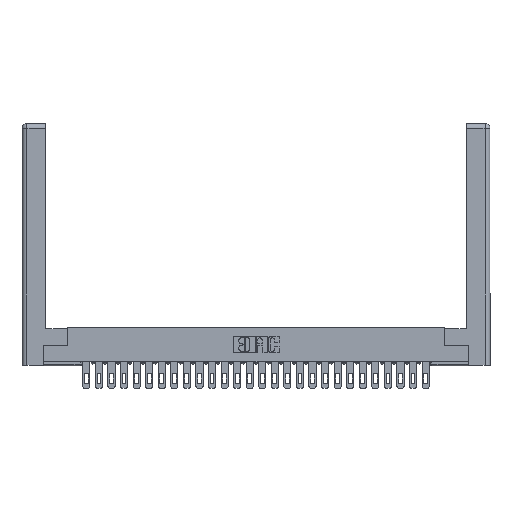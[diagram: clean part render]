
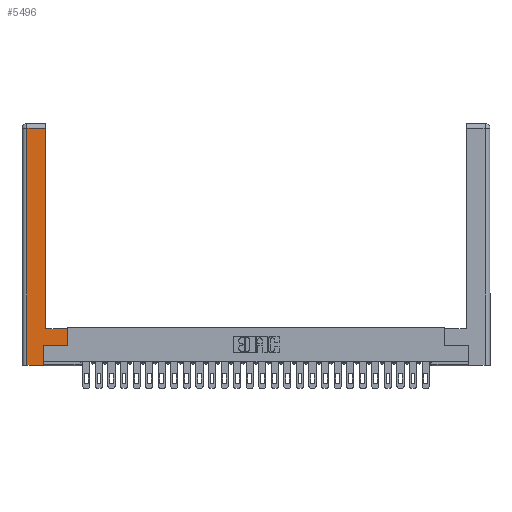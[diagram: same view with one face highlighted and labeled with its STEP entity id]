
A CAD part, top view. The second image highlights one B-rep face of the part: STEP entity #5496.
In plain terms, the highlighted planar face has unit normal (0, 0, 1).
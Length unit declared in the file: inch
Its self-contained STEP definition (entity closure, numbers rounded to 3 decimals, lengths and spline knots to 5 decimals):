
#522 = CARTESIAN_POINT ( 'NONE',  ( 0.295, 2.94, 0. ) ) ;
#1122 = CARTESIAN_POINT ( 'NONE',  ( 0.295, 3., 0. ) ) ;
#1353 = VECTOR ( 'NONE', #4804, 39.37008 ) ;
#2107 = VECTOR ( 'NONE', #16895, 39.37008 ) ;
#3837 = LINE ( 'NONE', #25675, #9139 ) ;
#3874 = PLANE ( 'NONE',  #5296 ) ;
#4760 = CARTESIAN_POINT ( 'NONE',  ( 0.265, 0., 0. ) ) ;
#4804 = DIRECTION ( 'NONE',  ( 0., 1., 0. ) ) ;
#4821 = VERTEX_POINT ( 'NONE', #28256 ) ;
#4866 = EDGE_CURVE ( 'NONE', #8910, #16377, #15898, .T. ) ;
#5296 = AXIS2_PLACEMENT_3D ( 'NONE', #28823, #24265, #22078 ) ;
#5496 = ADVANCED_FACE ( 'NONE', ( #17241 ), #3874, .F. ) ;
#6043 = VERTEX_POINT ( 'NONE', #23443 ) ;
#6126 = ORIENTED_EDGE ( 'NONE', *, *, #4866, .T. ) ;
#7914 = ORIENTED_EDGE ( 'NONE', *, *, #8423, .T. ) ;
#8423 = EDGE_CURVE ( 'NONE', #4821, #15440, #24903, .T. ) ;
#8910 = VERTEX_POINT ( 'NONE', #12033 ) ;
#8972 = LINE ( 'NONE', #1122, #28034 ) ;
#9139 = VECTOR ( 'NONE', #23198, 39.37008 ) ;
#9192 = VERTEX_POINT ( 'NONE', #15165 ) ;
#9513 = LINE ( 'NONE', #21957, #22514 ) ;
#11246 = LINE ( 'NONE', #25083, #1353 ) ;
#11441 = LINE ( 'NONE', #4760, #25546 ) ;
#11671 = CARTESIAN_POINT ( 'NONE',  ( 0.265, 0.245, 0. ) ) ;
#11865 = EDGE_CURVE ( 'NONE', #12794, #25649, #9513, .T. ) ;
#12033 = CARTESIAN_POINT ( 'NONE',  ( 0.565, 0.45, 0. ) ) ;
#12794 = VERTEX_POINT ( 'NONE', #522 ) ;
#12939 = VECTOR ( 'NONE', #23481, 39.37008 ) ;
#15165 = CARTESIAN_POINT ( 'NONE',  ( 0.0615, 0., 0. ) ) ;
#15440 = VERTEX_POINT ( 'NONE', #20971 ) ;
#15492 = ORIENTED_EDGE ( 'NONE', *, *, #21818, .T. ) ;
#15898 = LINE ( 'NONE', #19530, #2107 ) ;
#16377 = VERTEX_POINT ( 'NONE', #22408 ) ;
#16895 = DIRECTION ( 'NONE',  ( -1., 0., 0. ) ) ;
#17241 = FACE_OUTER_BOUND ( 'NONE', #18652, .T. ) ;
#17528 = DIRECTION ( 'NONE',  ( -1., 0., 0. ) ) ;
#18396 = DIRECTION ( 'NONE',  ( 1., 0., 0. ) ) ;
#18652 = EDGE_LOOP ( 'NONE', ( #28800, #19707, #15492, #23686, #26910, #7914, #23091, #6126 ) ) ;
#18724 = EDGE_CURVE ( 'NONE', #9192, #6043, #11441, .T. ) ;
#19299 = VECTOR ( 'NONE', #20702, 39.37008 ) ;
#19530 = CARTESIAN_POINT ( 'NONE',  ( 0.295, 0.45, 0. ) ) ;
#19707 = ORIENTED_EDGE ( 'NONE', *, *, #11865, .T. ) ;
#20702 = DIRECTION ( 'NONE',  ( 0., 1., 0. ) ) ;
#20825 = CARTESIAN_POINT ( 'NONE',  ( 0.0615, 2.94, 0. ) ) ;
#20971 = CARTESIAN_POINT ( 'NONE',  ( 0.565, 0.245, 0. ) ) ;
#21097 = CARTESIAN_POINT ( 'NONE',  ( 0.565, 0.245, 0. ) ) ;
#21429 = DIRECTION ( 'NONE',  ( 0., 1., 0. ) ) ;
#21697 = EDGE_CURVE ( 'NONE', #15440, #8910, #11246, .T. ) ;
#21759 = LINE ( 'NONE', #11671, #19299 ) ;
#21818 = EDGE_CURVE ( 'NONE', #25649, #9192, #3837, .T. ) ;
#21957 = CARTESIAN_POINT ( 'NONE',  ( 0.0615, 2.94, 0. ) ) ;
#22078 = DIRECTION ( 'NONE',  ( -1., 0., 0. ) ) ;
#22408 = CARTESIAN_POINT ( 'NONE',  ( 0.295, 0.45, 0. ) ) ;
#22514 = VECTOR ( 'NONE', #17528, 39.37008 ) ;
#23091 = ORIENTED_EDGE ( 'NONE', *, *, #21697, .T. ) ;
#23198 = DIRECTION ( 'NONE',  ( 0., -1., 0. ) ) ;
#23408 = EDGE_CURVE ( 'NONE', #6043, #4821, #21759, .T. ) ;
#23443 = CARTESIAN_POINT ( 'NONE',  ( 0.265, 0., 0. ) ) ;
#23481 = DIRECTION ( 'NONE',  ( 1., 0., 0. ) ) ;
#23686 = ORIENTED_EDGE ( 'NONE', *, *, #18724, .T. ) ;
#24265 = DIRECTION ( 'NONE',  ( 0., 0., -1. ) ) ;
#24903 = LINE ( 'NONE', #21097, #12939 ) ;
#25083 = CARTESIAN_POINT ( 'NONE',  ( 0.565, 0.45, 0. ) ) ;
#25546 = VECTOR ( 'NONE', #18396, 39.37008 ) ;
#25649 = VERTEX_POINT ( 'NONE', #20825 ) ;
#25675 = CARTESIAN_POINT ( 'NONE',  ( 0.0615, 0., 0. ) ) ;
#25845 = EDGE_CURVE ( 'NONE', #16377, #12794, #8972, .T. ) ;
#26910 = ORIENTED_EDGE ( 'NONE', *, *, #23408, .T. ) ;
#28034 = VECTOR ( 'NONE', #21429, 39.37008 ) ;
#28256 = CARTESIAN_POINT ( 'NONE',  ( 0.265, 0.245, 0. ) ) ;
#28800 = ORIENTED_EDGE ( 'NONE', *, *, #25845, .T. ) ;
#28823 = CARTESIAN_POINT ( 'NONE',  ( 0., 0., 0. ) ) ;
